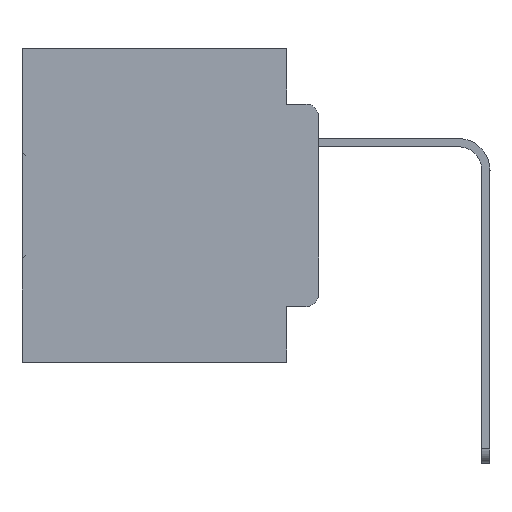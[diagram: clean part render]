
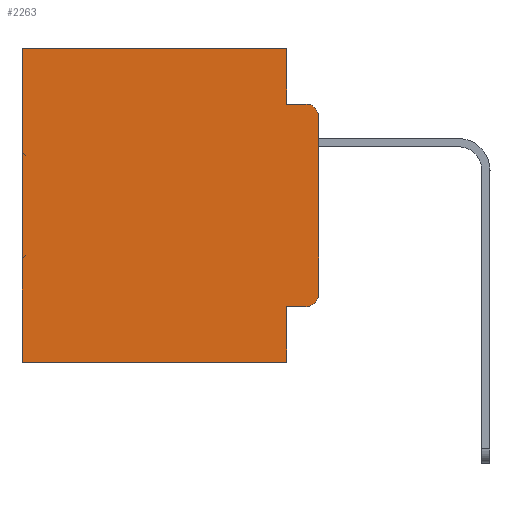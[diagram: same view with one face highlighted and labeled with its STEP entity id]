
A CAD part, left-side view. The second image highlights one B-rep face of the part: STEP entity #2263.
In plain terms, the highlighted planar face has unit normal (-1, 0, 0).
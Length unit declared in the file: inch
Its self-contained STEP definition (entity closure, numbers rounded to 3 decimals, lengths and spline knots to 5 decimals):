
#424 = VERTEX_POINT ( 'NONE', #7626 ) ;
#444 = VECTOR ( 'NONE', #15262, 39.37008 ) ;
#478 = VECTOR ( 'NONE', #23326, 39.37008 ) ;
#1478 = EDGE_CURVE ( 'NONE', #22277, #14803, #33932, .T. ) ;
#1500 = CARTESIAN_POINT ( 'NONE',  ( 0.298, 0.02, -0.3915 ) ) ;
#2130 = CARTESIAN_POINT ( 'NONE',  ( 0.298, 0.051, -0.0885 ) ) ;
#2258 = ORIENTED_EDGE ( 'NONE', *, *, #27724, .T. ) ;
#2263 = ADVANCED_FACE ( 'NONE', ( #17683 ), #21129, .F. ) ;
#3485 = ORIENTED_EDGE ( 'NONE', *, *, #1478, .F. ) ;
#3657 = CIRCLE ( 'NONE', #10242, 0.02 ) ;
#5197 = CARTESIAN_POINT ( 'NONE',  ( 0.298, 0.473, 0. ) ) ;
#5407 = EDGE_CURVE ( 'NONE', #7100, #8643, #15297, .T. ) ;
#5708 = DIRECTION ( 'NONE',  ( 0., 0., -1. ) ) ;
#6860 = EDGE_CURVE ( 'NONE', #10129, #8643, #25503, .T. ) ;
#7100 = VERTEX_POINT ( 'NONE', #19504 ) ;
#7408 = EDGE_CURVE ( 'NONE', #25417, #33979, #19193, .T. ) ;
#7505 = CARTESIAN_POINT ( 'NONE',  ( 0.298, 0.02, -0.1085 ) ) ;
#7626 = CARTESIAN_POINT ( 'NONE',  ( 0.298, 0.02, -0.0885 ) ) ;
#7625 = DIRECTION ( 'NONE',  ( 0., 0., -1. ) ) ;
#7736 = VECTOR ( 'NONE', #5708, 39.37008 ) ;
#8137 = ORIENTED_EDGE ( 'NONE', *, *, #15434, .T. ) ;
#8643 = VERTEX_POINT ( 'NONE', #16797 ) ;
#9470 = EDGE_CURVE ( 'NONE', #25288, #13878, #20744, .T. ) ;
#9562 = AXIS2_PLACEMENT_3D ( 'NONE', #29348, #13484, #32025 ) ;
#9771 = CARTESIAN_POINT ( 'NONE',  ( 0.298, 0.051, 0. ) ) ;
#10129 = VERTEX_POINT ( 'NONE', #19798 ) ;
#10242 = AXIS2_PLACEMENT_3D ( 'NONE', #7505, #28828, #7625 ) ;
#10709 = DIRECTION ( 'NONE',  ( 0., 0., -1. ) ) ;
#11168 = CARTESIAN_POINT ( 'NONE',  ( 0.298, 0.02, -0.4115 ) ) ;
#12357 = DIRECTION ( 'NONE',  ( 0., 1., 0. ) ) ;
#12416 = LINE ( 'NONE', #25997, #32336 ) ;
#12428 = DIRECTION ( 'NONE',  ( 0., 0., -1. ) ) ;
#12578 = CARTESIAN_POINT ( 'NONE',  ( 0.298, 0.051, -0.0885 ) ) ;
#12780 = VECTOR ( 'NONE', #12357, 39.37008 ) ;
#13388 = AXIS2_PLACEMENT_3D ( 'NONE', #1500, #20292, #12428 ) ;
#13484 = DIRECTION ( 'NONE',  ( 1., 0., 0. ) ) ;
#13878 = VERTEX_POINT ( 'NONE', #14166 ) ;
#13963 = EDGE_CURVE ( 'NONE', #33979, #13878, #31190, .T. ) ;
#14166 = CARTESIAN_POINT ( 'NONE',  ( 0.298, 0., -0.3915 ) ) ;
#14532 = CARTESIAN_POINT ( 'NONE',  ( 0.298, 0., 0. ) ) ;
#14803 = VERTEX_POINT ( 'NONE', #2130 ) ;
#14958 = LINE ( 'NONE', #9771, #478 ) ;
#15262 = DIRECTION ( 'NONE',  ( 0., -1., 0. ) ) ;
#15270 = EDGE_CURVE ( 'NONE', #25417, #7100, #14958, .T. ) ;
#15297 = LINE ( 'NONE', #33939, #12780 ) ;
#15342 = CARTESIAN_POINT ( 'NONE',  ( 0.298, 0., -0.1085 ) ) ;
#15434 = EDGE_CURVE ( 'NONE', #22277, #10129, #12416, .T. ) ;
#16590 = ORIENTED_EDGE ( 'NONE', *, *, #5407, .F. ) ;
#16797 = CARTESIAN_POINT ( 'NONE',  ( 0.298, 0.473, -0.5 ) ) ;
#17683 = FACE_OUTER_BOUND ( 'NONE', #18114, .T. ) ;
#18113 = DIRECTION ( 'NONE',  ( 0., -1., 0. ) ) ;
#18114 = EDGE_LOOP ( 'NONE', ( #26584, #2258, #22663, #3485, #8137, #28642, #16590, #18277, #32970, #30782 ) ) ;
#18277 = ORIENTED_EDGE ( 'NONE', *, *, #15270, .F. ) ;
#18431 = VECTOR ( 'NONE', #10709, 39.37008 ) ;
#18569 = DIRECTION ( 'NONE',  ( 0., 1., 0. ) ) ;
#19193 = LINE ( 'NONE', #31199, #26665 ) ;
#19504 = CARTESIAN_POINT ( 'NONE',  ( 0.298, 0.051, -0.5 ) ) ;
#19798 = CARTESIAN_POINT ( 'NONE',  ( 0.298, 0.473, 0. ) ) ;
#20292 = DIRECTION ( 'NONE',  ( -1., 0., 0. ) ) ;
#20744 = LINE ( 'NONE', #14532, #32391 ) ;
#21102 = CARTESIAN_POINT ( 'NONE',  ( 0.298, 0.051, -0.4115 ) ) ;
#21129 = PLANE ( 'NONE',  #9562 ) ;
#22277 = VERTEX_POINT ( 'NONE', #28847 ) ;
#22663 = ORIENTED_EDGE ( 'NONE', *, *, #26558, .F. ) ;
#23326 = DIRECTION ( 'NONE',  ( 0., 0., -1. ) ) ;
#24208 = CARTESIAN_POINT ( 'NONE',  ( 0.298, 0.051, 0. ) ) ;
#25288 = VERTEX_POINT ( 'NONE', #15342 ) ;
#25417 = VERTEX_POINT ( 'NONE', #21102 ) ;
#25503 = LINE ( 'NONE', #5197, #18431 ) ;
#25997 = CARTESIAN_POINT ( 'NONE',  ( 0.298, 0., 0. ) ) ;
#26502 = LINE ( 'NONE', #12578, #444 ) ;
#26558 = EDGE_CURVE ( 'NONE', #14803, #424, #26502, .T. ) ;
#26584 = ORIENTED_EDGE ( 'NONE', *, *, #9470, .F. ) ;
#26665 = VECTOR ( 'NONE', #18113, 39.37008 ) ;
#27472 = DIRECTION ( 'NONE',  ( 0., 0., -1. ) ) ;
#27724 = EDGE_CURVE ( 'NONE', #25288, #424, #3657, .T. ) ;
#28642 = ORIENTED_EDGE ( 'NONE', *, *, #6860, .T. ) ;
#28828 = DIRECTION ( 'NONE',  ( -1., 0., 0. ) ) ;
#28847 = CARTESIAN_POINT ( 'NONE',  ( 0.298, 0.051, 0. ) ) ;
#29348 = CARTESIAN_POINT ( 'NONE',  ( 0.298, 0., 0. ) ) ;
#30782 = ORIENTED_EDGE ( 'NONE', *, *, #13963, .T. ) ;
#31190 = CIRCLE ( 'NONE', #13388, 0.02 ) ;
#31199 = CARTESIAN_POINT ( 'NONE',  ( 0.298, 0.051, -0.4115 ) ) ;
#32025 = DIRECTION ( 'NONE',  ( 0., 0., -1. ) ) ;
#32336 = VECTOR ( 'NONE', #18569, 39.37008 ) ;
#32391 = VECTOR ( 'NONE', #27472, 39.37008 ) ;
#32970 = ORIENTED_EDGE ( 'NONE', *, *, #7408, .T. ) ;
#33932 = LINE ( 'NONE', #24208, #7736 ) ;
#33939 = CARTESIAN_POINT ( 'NONE',  ( 0.298, 0., -0.5 ) ) ;
#33979 = VERTEX_POINT ( 'NONE', #11168 ) ;
